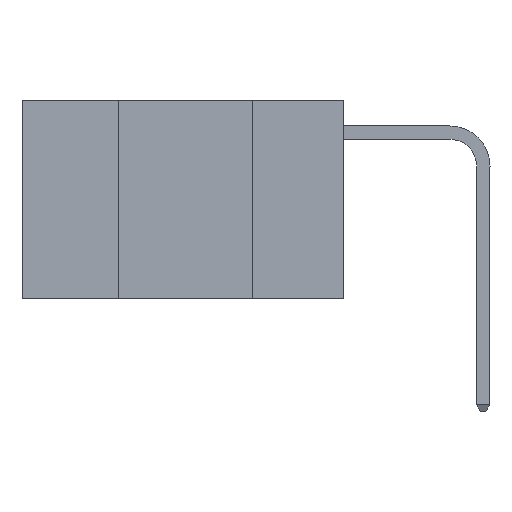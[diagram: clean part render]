
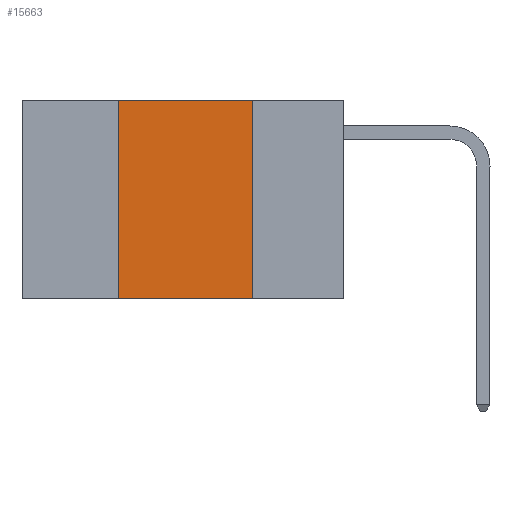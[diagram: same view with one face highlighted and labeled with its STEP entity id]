
A CAD part, left-side view. The second image highlights one B-rep face of the part: STEP entity #15663.
In plain terms, the highlighted planar face has unit normal (-1, 0, 0).
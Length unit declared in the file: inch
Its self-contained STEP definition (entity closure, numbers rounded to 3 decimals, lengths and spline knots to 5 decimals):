
#1310 = DIRECTION ( 'NONE',  ( 1., 0., 0. ) ) ;
#2545 = CARTESIAN_POINT ( 'NONE',  ( 0., 0.17, 0. ) ) ;
#2626 = LINE ( 'NONE', #11751, #13676 ) ;
#2664 = LINE ( 'NONE', #10263, #11795 ) ;
#2998 = VERTEX_POINT ( 'NONE', #8098 ) ;
#3045 = ORIENTED_EDGE ( 'NONE', *, *, #10765, .F. ) ;
#3154 = ORIENTED_EDGE ( 'NONE', *, *, #7655, .F. ) ;
#3200 = ORIENTED_EDGE ( 'NONE', *, *, #9942, .F. ) ;
#3373 = ORIENTED_EDGE ( 'NONE', *, *, #9091, .T. ) ;
#4305 = DIRECTION ( 'NONE',  ( 0., -1., 0. ) ) ;
#4391 = DIRECTION ( 'NONE',  ( 0., 0., 1. ) ) ;
#4738 = VERTEX_POINT ( 'NONE', #6483 ) ;
#5096 = CARTESIAN_POINT ( 'NONE',  ( 0., 0.42, -0.37 ) ) ;
#6339 = VERTEX_POINT ( 'NONE', #5096 ) ;
#6483 = CARTESIAN_POINT ( 'NONE',  ( 0., 0.17, -0.37 ) ) ;
#7494 = DIRECTION ( 'NONE',  ( 0., 0., -1. ) ) ;
#7655 = EDGE_CURVE ( 'NONE', #2998, #14539, #2664, .T. ) ;
#8098 = CARTESIAN_POINT ( 'NONE',  ( 0., 0.42, 0. ) ) ;
#8360 = FACE_OUTER_BOUND ( 'NONE', #10635, .T. ) ;
#8871 = CARTESIAN_POINT ( 'NONE',  ( 0., 0.6, 0. ) ) ;
#9091 = EDGE_CURVE ( 'NONE', #6339, #4738, #2626, .T. ) ;
#9157 = VECTOR ( 'NONE', #7494, 39.37008 ) ;
#9372 = LINE ( 'NONE', #13067, #9761 ) ;
#9761 = VECTOR ( 'NONE', #4391, 39.37008 ) ;
#9942 = EDGE_CURVE ( 'NONE', #6339, #2998, #9372, .T. ) ;
#10112 = DIRECTION ( 'NONE',  ( 0., 0., -1. ) ) ;
#10263 = CARTESIAN_POINT ( 'NONE',  ( 0., 0.6, 0. ) ) ;
#10635 = EDGE_LOOP ( 'NONE', ( #3045, #3154, #3200, #3373 ) ) ;
#10765 = EDGE_CURVE ( 'NONE', #14539, #4738, #12521, .T. ) ;
#11751 = CARTESIAN_POINT ( 'NONE',  ( 0., 0.6, -0.37 ) ) ;
#11795 = VECTOR ( 'NONE', #13965, 39.37008 ) ;
#12521 = LINE ( 'NONE', #15958, #9157 ) ;
#13067 = CARTESIAN_POINT ( 'NONE',  ( 0., 0.42, 0. ) ) ;
#13676 = VECTOR ( 'NONE', #4305, 39.37008 ) ;
#13736 = PLANE ( 'NONE',  #14241 ) ;
#13965 = DIRECTION ( 'NONE',  ( 0., -1., 0. ) ) ;
#14241 = AXIS2_PLACEMENT_3D ( 'NONE', #8871, #1310, #10112 ) ;
#14539 = VERTEX_POINT ( 'NONE', #2545 ) ;
#15663 = ADVANCED_FACE ( 'NONE', ( #8360 ), #13736, .F. ) ;
#15958 = CARTESIAN_POINT ( 'NONE',  ( 0., 0.17, 0. ) ) ;
